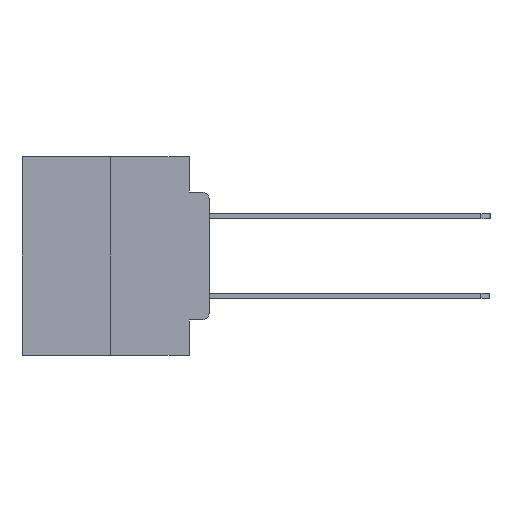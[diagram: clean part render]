
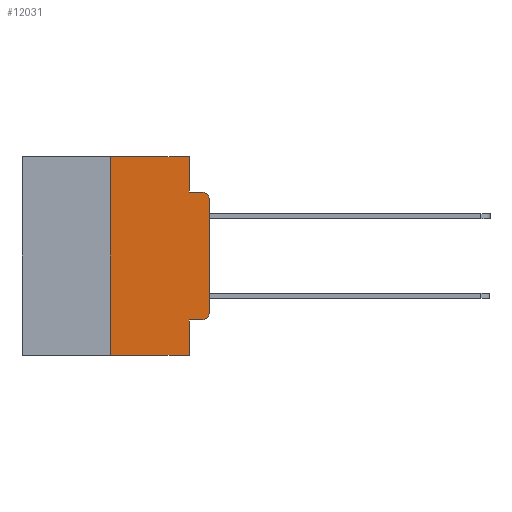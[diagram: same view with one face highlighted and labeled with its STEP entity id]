
A CAD part, left-side view. The second image highlights one B-rep face of the part: STEP entity #12031.
In plain terms, the highlighted planar face has unit normal (-1, 0, 0).
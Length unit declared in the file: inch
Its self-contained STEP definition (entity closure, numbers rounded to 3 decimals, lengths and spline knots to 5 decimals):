
#378 = EDGE_CURVE ( 'NONE', #11723, #14201, #5458, .T. ) ;
#776 = VECTOR ( 'NONE', #9288, 39.37008 ) ;
#953 = DIRECTION ( 'NONE',  ( 0., 0., -1. ) ) ;
#1141 = EDGE_CURVE ( 'NONE', #11965, #8309, #21664, .T. ) ;
#1459 = AXIS2_PLACEMENT_3D ( 'NONE', #27973, #15299, #2102 ) ;
#1711 = CARTESIAN_POINT ( 'NONE',  ( 0., 0., -0.1085 ) ) ;
#2102 = DIRECTION ( 'NONE',  ( 0., 0., -1. ) ) ;
#2777 = FACE_OUTER_BOUND ( 'NONE', #7154, .T. ) ;
#3178 = ORIENTED_EDGE ( 'NONE', *, *, #14856, .F. ) ;
#3312 = CARTESIAN_POINT ( 'NONE',  ( 0., 0.02, -0.3915 ) ) ;
#3328 = VERTEX_POINT ( 'NONE', #26693 ) ;
#3425 = EDGE_CURVE ( 'NONE', #8425, #11723, #27509, .T. ) ;
#3607 = CARTESIAN_POINT ( 'NONE',  ( 0., 0.02, -0.0885 ) ) ;
#3997 = CARTESIAN_POINT ( 'NONE',  ( 0., 0.473, 0. ) ) ;
#4571 = CARTESIAN_POINT ( 'NONE',  ( 0., 0.051, -0.0885 ) ) ;
#4626 = CARTESIAN_POINT ( 'NONE',  ( 0., 0.051, -0.5 ) ) ;
#4699 = VECTOR ( 'NONE', #13724, 39.37008 ) ;
#5390 = LINE ( 'NONE', #11572, #4699 ) ;
#5458 = LINE ( 'NONE', #12879, #17059 ) ;
#5556 = DIRECTION ( 'NONE',  ( 0., 0., -1. ) ) ;
#5855 = EDGE_CURVE ( 'NONE', #11965, #8425, #16989, .T. ) ;
#5879 = EDGE_CURVE ( 'NONE', #23438, #3328, #5390, .T. ) ;
#6211 = DIRECTION ( 'NONE',  ( 0., -1., 0. ) ) ;
#6219 = DIRECTION ( 'NONE',  ( 0., 0., -1. ) ) ;
#6976 = EDGE_CURVE ( 'NONE', #14201, #11173, #22890, .T. ) ;
#7154 = EDGE_LOOP ( 'NONE', ( #9446, #22850, #3178, #14881, #26145, #26815, #11164, #20215, #10165, #21562 ) ) ;
#8309 = VERTEX_POINT ( 'NONE', #4626 ) ;
#8425 = VERTEX_POINT ( 'NONE', #18041 ) ;
#9288 = DIRECTION ( 'NONE',  ( 0., -1., 0. ) ) ;
#9446 = ORIENTED_EDGE ( 'NONE', *, *, #378, .T. ) ;
#10165 = ORIENTED_EDGE ( 'NONE', *, *, #5855, .T. ) ;
#10257 = VECTOR ( 'NONE', #23320, 39.37008 ) ;
#11055 = EDGE_CURVE ( 'NONE', #24165, #23438, #13018, .T. ) ;
#11090 = AXIS2_PLACEMENT_3D ( 'NONE', #3312, #18564, #5556 ) ;
#11164 = ORIENTED_EDGE ( 'NONE', *, *, #27877, .T. ) ;
#11173 = VERTEX_POINT ( 'NONE', #3607 ) ;
#11572 = CARTESIAN_POINT ( 'NONE',  ( 0., 0.473, 0. ) ) ;
#11723 = VERTEX_POINT ( 'NONE', #15683 ) ;
#11772 = VECTOR ( 'NONE', #953, 39.37008 ) ;
#11821 = CARTESIAN_POINT ( 'NONE',  ( 0., 0.25, -0.5 ) ) ;
#11965 = VERTEX_POINT ( 'NONE', #25301 ) ;
#12007 = DIRECTION ( 'NONE',  ( 0., 0., 1. ) ) ;
#12031 = ADVANCED_FACE ( 'NONE', ( #2777 ), #12730, .F. ) ;
#12730 = PLANE ( 'NONE',  #16667 ) ;
#12879 = CARTESIAN_POINT ( 'NONE',  ( 0., 0., 0. ) ) ;
#13018 = LINE ( 'NONE', #16337, #17404 ) ;
#13037 = DIRECTION ( 'NONE',  ( 0., 0., 1. ) ) ;
#13724 = DIRECTION ( 'NONE',  ( 0., -1., 0. ) ) ;
#14201 = VERTEX_POINT ( 'NONE', #1711 ) ;
#14411 = DIRECTION ( 'NONE',  ( 0., 0., -1. ) ) ;
#14856 = EDGE_CURVE ( 'NONE', #26887, #11173, #26585, .T. ) ;
#14881 = ORIENTED_EDGE ( 'NONE', *, *, #17534, .F. ) ;
#15299 = DIRECTION ( 'NONE',  ( -1., 0., 0. ) ) ;
#15683 = CARTESIAN_POINT ( 'NONE',  ( 0., 0., -0.3915 ) ) ;
#16337 = CARTESIAN_POINT ( 'NONE',  ( 0., 0.25, 0. ) ) ;
#16667 = AXIS2_PLACEMENT_3D ( 'NONE', #3997, #19185, #6219 ) ;
#16989 = LINE ( 'NONE', #22123, #776 ) ;
#17059 = VECTOR ( 'NONE', #13037, 39.37008 ) ;
#17404 = VECTOR ( 'NONE', #12007, 39.37008 ) ;
#17499 = LINE ( 'NONE', #24818, #11772 ) ;
#17534 = EDGE_CURVE ( 'NONE', #3328, #26887, #17499, .T. ) ;
#18041 = CARTESIAN_POINT ( 'NONE',  ( 0., 0.02, -0.4115 ) ) ;
#18564 = DIRECTION ( 'NONE',  ( -1., 0., 0. ) ) ;
#19185 = DIRECTION ( 'NONE',  ( 1., 0., 0. ) ) ;
#19810 = LINE ( 'NONE', #21235, #24794 ) ;
#20215 = ORIENTED_EDGE ( 'NONE', *, *, #1141, .F. ) ;
#21235 = CARTESIAN_POINT ( 'NONE',  ( 0., 0.473, -0.5 ) ) ;
#21562 = ORIENTED_EDGE ( 'NONE', *, *, #3425, .T. ) ;
#21664 = LINE ( 'NONE', #27603, #27261 ) ;
#22123 = CARTESIAN_POINT ( 'NONE',  ( 0., 0.051, -0.4115 ) ) ;
#22850 = ORIENTED_EDGE ( 'NONE', *, *, #6976, .T. ) ;
#22890 = CIRCLE ( 'NONE', #1459, 0.02 ) ;
#23320 = DIRECTION ( 'NONE',  ( 0., -1., 0. ) ) ;
#23438 = VERTEX_POINT ( 'NONE', #23799 ) ;
#23799 = CARTESIAN_POINT ( 'NONE',  ( 0., 0.25, 0. ) ) ;
#24165 = VERTEX_POINT ( 'NONE', #11821 ) ;
#24794 = VECTOR ( 'NONE', #6211, 39.37008 ) ;
#24818 = CARTESIAN_POINT ( 'NONE',  ( 0., 0.051, 0. ) ) ;
#25301 = CARTESIAN_POINT ( 'NONE',  ( 0., 0.051, -0.4115 ) ) ;
#26145 = ORIENTED_EDGE ( 'NONE', *, *, #5879, .F. ) ;
#26585 = LINE ( 'NONE', #27467, #10257 ) ;
#26693 = CARTESIAN_POINT ( 'NONE',  ( 0., 0.051, 0. ) ) ;
#26815 = ORIENTED_EDGE ( 'NONE', *, *, #11055, .F. ) ;
#26887 = VERTEX_POINT ( 'NONE', #4571 ) ;
#27261 = VECTOR ( 'NONE', #14411, 39.37008 ) ;
#27467 = CARTESIAN_POINT ( 'NONE',  ( 0., 0.051, -0.0885 ) ) ;
#27509 = CIRCLE ( 'NONE', #11090, 0.02 ) ;
#27603 = CARTESIAN_POINT ( 'NONE',  ( 0., 0.051, 0. ) ) ;
#27877 = EDGE_CURVE ( 'NONE', #24165, #8309, #19810, .T. ) ;
#27973 = CARTESIAN_POINT ( 'NONE',  ( 0., 0.02, -0.1085 ) ) ;
